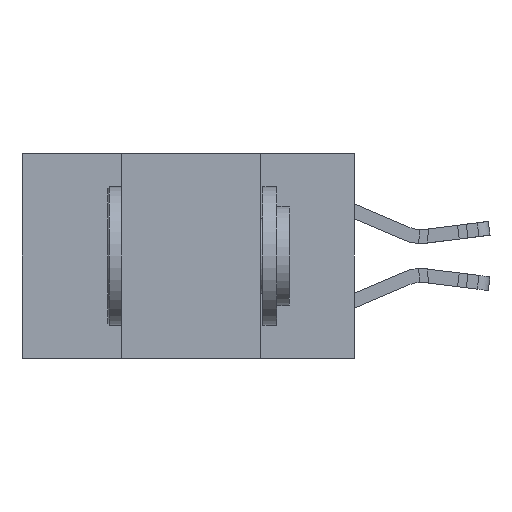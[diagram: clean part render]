
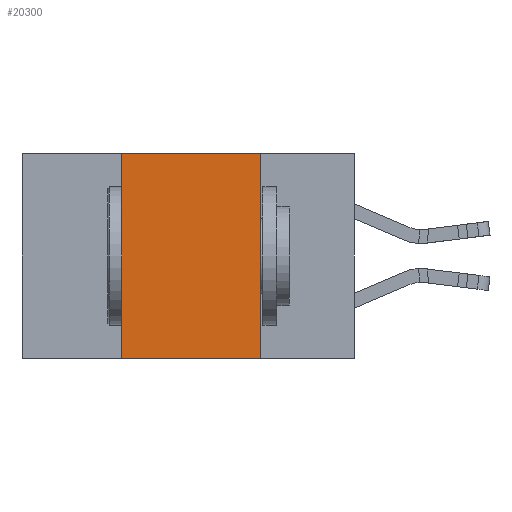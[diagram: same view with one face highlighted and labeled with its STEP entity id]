
A CAD part, left-side view. The second image highlights one B-rep face of the part: STEP entity #20300.
In plain terms, the highlighted planar face has unit normal (-1, 0, 0).
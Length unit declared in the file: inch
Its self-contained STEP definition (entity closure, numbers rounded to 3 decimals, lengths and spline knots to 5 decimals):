
#245 = VECTOR ( 'NONE', #14288, 39.37008 ) ;
#1208 = CARTESIAN_POINT ( 'NONE',  ( 0., 0.6, -0.37 ) ) ;
#2828 = EDGE_CURVE ( 'NONE', #12553, #17524, #20964, .T. ) ;
#4446 = LINE ( 'NONE', #16629, #245 ) ;
#5029 = CARTESIAN_POINT ( 'NONE',  ( 0., 0.17, -0.37 ) ) ;
#6391 = LINE ( 'NONE', #14289, #15341 ) ;
#6934 = ORIENTED_EDGE ( 'NONE', *, *, #13919, .F. ) ;
#7527 = FACE_OUTER_BOUND ( 'NONE', #21788, .T. ) ;
#9975 = VECTOR ( 'NONE', #12714, 39.37008 ) ;
#9981 = CARTESIAN_POINT ( 'NONE',  ( 0., 0.6, 0. ) ) ;
#10975 = DIRECTION ( 'NONE',  ( 0., 0., -1. ) ) ;
#12553 = VERTEX_POINT ( 'NONE', #13247 ) ;
#12714 = DIRECTION ( 'NONE',  ( 0., -1., 0. ) ) ;
#13247 = CARTESIAN_POINT ( 'NONE',  ( 0., 0.17, 0. ) ) ;
#13745 = CARTESIAN_POINT ( 'NONE',  ( 0., 0.17, -0.37 ) ) ;
#13919 = EDGE_CURVE ( 'NONE', #25522, #14048, #4446, .T. ) ;
#14048 = VERTEX_POINT ( 'NONE', #15045 ) ;
#14288 = DIRECTION ( 'NONE',  ( 0., 0., 1. ) ) ;
#14289 = CARTESIAN_POINT ( 'NONE',  ( 0., 0.6, 0. ) ) ;
#15045 = CARTESIAN_POINT ( 'NONE',  ( 0., 0.42, 0. ) ) ;
#15341 = VECTOR ( 'NONE', #22204, 39.37008 ) ;
#15689 = PLANE ( 'NONE',  #23575 ) ;
#15830 = ORIENTED_EDGE ( 'NONE', *, *, #2828, .F. ) ;
#16629 = CARTESIAN_POINT ( 'NONE',  ( 0., 0.42, -0.37 ) ) ;
#17524 = VERTEX_POINT ( 'NONE', #13745 ) ;
#18948 = LINE ( 'NONE', #1208, #9975 ) ;
#19585 = DIRECTION ( 'NONE',  ( 0., 0., -1. ) ) ;
#20243 = ORIENTED_EDGE ( 'NONE', *, *, #22350, .F. ) ;
#20300 = ADVANCED_FACE ( 'NONE', ( #7527 ), #15689, .F. ) ;
#20964 = LINE ( 'NONE', #5029, #22180 ) ;
#21255 = CARTESIAN_POINT ( 'NONE',  ( 0., 0.42, -0.37 ) ) ;
#21785 = DIRECTION ( 'NONE',  ( 1., 0., 0. ) ) ;
#21788 = EDGE_LOOP ( 'NONE', ( #15830, #20243, #6934, #24168 ) ) ;
#22180 = VECTOR ( 'NONE', #10975, 39.37008 ) ;
#22204 = DIRECTION ( 'NONE',  ( 0., -1., 0. ) ) ;
#22350 = EDGE_CURVE ( 'NONE', #14048, #12553, #6391, .T. ) ;
#22462 = EDGE_CURVE ( 'NONE', #25522, #17524, #18948, .T. ) ;
#23575 = AXIS2_PLACEMENT_3D ( 'NONE', #9981, #21785, #19585 ) ;
#24168 = ORIENTED_EDGE ( 'NONE', *, *, #22462, .T. ) ;
#25522 = VERTEX_POINT ( 'NONE', #21255 ) ;
